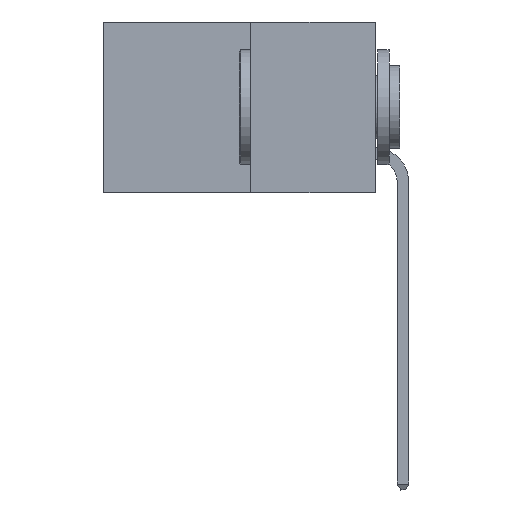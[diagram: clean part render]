
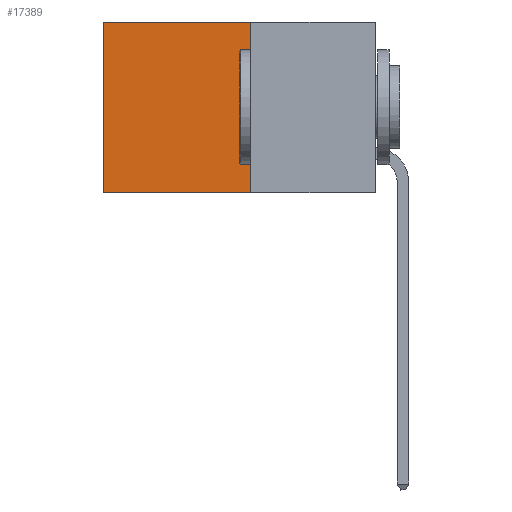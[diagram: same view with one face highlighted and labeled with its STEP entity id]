
A CAD part, left-side view. The second image highlights one B-rep face of the part: STEP entity #17389.
In plain terms, the highlighted planar face has unit normal (-1, 0, 0).
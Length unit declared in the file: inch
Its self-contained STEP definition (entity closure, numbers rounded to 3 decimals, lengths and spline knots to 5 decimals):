
#97 = VERTEX_POINT ( 'NONE', #8710 ) ;
#308 = LINE ( 'NONE', #2494, #10109 ) ;
#774 = DIRECTION ( 'NONE',  ( 0., 1., 0. ) ) ;
#1449 = CARTESIAN_POINT ( 'NONE',  ( 0.277, 0.27, 0. ) ) ;
#2494 = CARTESIAN_POINT ( 'NONE',  ( 0.277, 0.27, -0.37 ) ) ;
#2836 = CARTESIAN_POINT ( 'NONE',  ( 0.277, 0.27, 0. ) ) ;
#3300 = VECTOR ( 'NONE', #24785, 39.37008 ) ;
#3537 = PLANE ( 'NONE',  #23955 ) ;
#3582 = CARTESIAN_POINT ( 'NONE',  ( 0.277, 0.59, -0.37 ) ) ;
#3906 = LINE ( 'NONE', #25115, #3300 ) ;
#4432 = DIRECTION ( 'NONE',  ( 0., 0., -1. ) ) ;
#5479 = DIRECTION ( 'NONE',  ( 1., 0., 0. ) ) ;
#5511 = EDGE_CURVE ( 'NONE', #9486, #10686, #9724, .T. ) ;
#5533 = EDGE_CURVE ( 'NONE', #7169, #97, #3906, .T. ) ;
#6538 = ORIENTED_EDGE ( 'NONE', *, *, #5533, .F. ) ;
#7169 = VERTEX_POINT ( 'NONE', #23922 ) ;
#8710 = CARTESIAN_POINT ( 'NONE',  ( 0.277, 0.59, -0.37 ) ) ;
#9091 = CARTESIAN_POINT ( 'NONE',  ( 0.277, 0.59, 0. ) ) ;
#9317 = EDGE_LOOP ( 'NONE', ( #19385, #6538, #24105, #16399 ) ) ;
#9486 = VERTEX_POINT ( 'NONE', #2836 ) ;
#9724 = LINE ( 'NONE', #1449, #24725 ) ;
#10109 = VECTOR ( 'NONE', #4432, 39.37008 ) ;
#10686 = VERTEX_POINT ( 'NONE', #9091 ) ;
#15221 = VECTOR ( 'NONE', #19274, 39.37008 ) ;
#16399 = ORIENTED_EDGE ( 'NONE', *, *, #5511, .T. ) ;
#17274 = CARTESIAN_POINT ( 'NONE',  ( 0.277, 0.27, -0.37 ) ) ;
#17389 = ADVANCED_FACE ( 'NONE', ( #24250 ), #3537, .F. ) ;
#18372 = EDGE_CURVE ( 'NONE', #9486, #7169, #308, .T. ) ;
#19226 = DIRECTION ( 'NONE',  ( 0., 0., -1. ) ) ;
#19274 = DIRECTION ( 'NONE',  ( 0., 0., -1. ) ) ;
#19385 = ORIENTED_EDGE ( 'NONE', *, *, #21779, .T. ) ;
#20423 = LINE ( 'NONE', #3582, #15221 ) ;
#21779 = EDGE_CURVE ( 'NONE', #10686, #97, #20423, .T. ) ;
#23922 = CARTESIAN_POINT ( 'NONE',  ( 0.277, 0.27, -0.37 ) ) ;
#23955 = AXIS2_PLACEMENT_3D ( 'NONE', #17274, #5479, #19226 ) ;
#24105 = ORIENTED_EDGE ( 'NONE', *, *, #18372, .F. ) ;
#24250 = FACE_OUTER_BOUND ( 'NONE', #9317, .T. ) ;
#24725 = VECTOR ( 'NONE', #774, 39.37008 ) ;
#24785 = DIRECTION ( 'NONE',  ( 0., 1., 0. ) ) ;
#25115 = CARTESIAN_POINT ( 'NONE',  ( 0.277, 0.27, -0.37 ) ) ;
